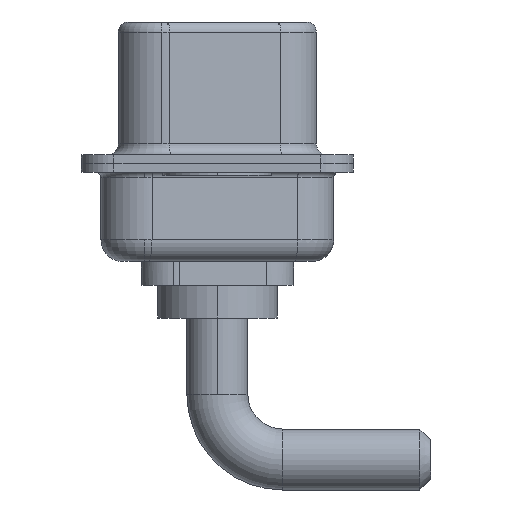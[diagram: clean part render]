
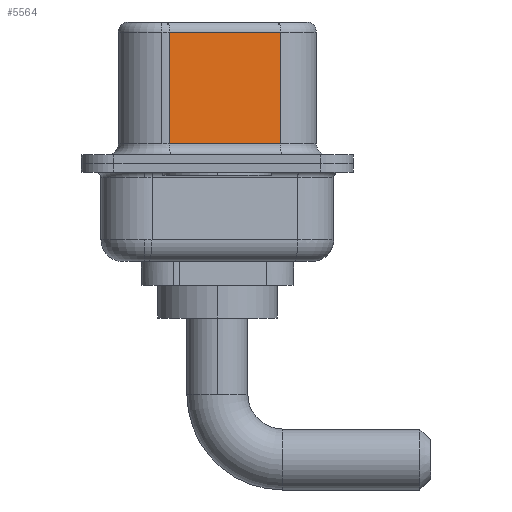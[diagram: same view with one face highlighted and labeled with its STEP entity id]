
A CAD part, left-side view. The second image highlights one B-rep face of the part: STEP entity #5564.
In plain terms, the highlighted planar face has unit normal (-0.985, -0.174, 0).
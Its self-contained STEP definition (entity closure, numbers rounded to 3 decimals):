
#86 = VECTOR ( 'NONE', #13597, 1000. ) ;
#564 = CARTESIAN_POINT ( 'NONE',  ( 3.68, 2.203, 6.02 ) ) ;
#1010 = DIRECTION ( 'NONE',  ( 0.174, -0.985, 0. ) ) ;
#1036 = EDGE_LOOP ( 'NONE', ( #1470, #6937, #10099, #8384 ) ) ;
#1463 = FACE_OUTER_BOUND ( 'NONE', #1036, .T. ) ;
#1470 = ORIENTED_EDGE ( 'NONE', *, *, #13379, .F. ) ;
#1583 = LINE ( 'NONE', #5954, #86 ) ;
#2079 = VECTOR ( 'NONE', #6700, 1000. ) ;
#2290 = CARTESIAN_POINT ( 'NONE',  ( 4.58, -2.897, 0.9 ) ) ;
#2529 = CARTESIAN_POINT ( 'NONE',  ( 4.58, -2.897, 6.52 ) ) ;
#2664 = LINE ( 'NONE', #5741, #14234 ) ;
#2770 = EDGE_CURVE ( 'NONE', #6604, #4736, #1583, .T. ) ;
#3302 = LINE ( 'NONE', #2290, #7508 ) ;
#3891 = EDGE_CURVE ( 'NONE', #5021, #6604, #4998, .T. ) ;
#4736 = VERTEX_POINT ( 'NONE', #10862 ) ;
#4998 = LINE ( 'NONE', #13854, #2079 ) ;
#5021 = VERTEX_POINT ( 'NONE', #9100 ) ;
#5564 = ADVANCED_FACE ( 'NONE', ( #1463 ), #5755, .F. ) ;
#5741 = CARTESIAN_POINT ( 'NONE',  ( 4.58, -2.897, 6.52 ) ) ;
#5755 = PLANE ( 'NONE',  #11990 ) ;
#5835 = DIRECTION ( 'NONE',  ( 0.985, 0.174, 0. ) ) ;
#5954 = CARTESIAN_POINT ( 'NONE',  ( 3.68, 2.203, 6.52 ) ) ;
#6604 = VERTEX_POINT ( 'NONE', #564 ) ;
#6700 = DIRECTION ( 'NONE',  ( -0.174, 0.985, 0. ) ) ;
#6937 = ORIENTED_EDGE ( 'NONE', *, *, #3891, .T. ) ;
#7508 = VECTOR ( 'NONE', #1010, 1000. ) ;
#8384 = ORIENTED_EDGE ( 'NONE', *, *, #13764, .T. ) ;
#9100 = CARTESIAN_POINT ( 'NONE',  ( 4.58, -2.897, 6.02 ) ) ;
#10099 = ORIENTED_EDGE ( 'NONE', *, *, #2770, .T. ) ;
#10308 = DIRECTION ( 'NONE',  ( -0.174, 0.985, 0. ) ) ;
#10862 = CARTESIAN_POINT ( 'NONE',  ( 3.68, 2.203, 0.9 ) ) ;
#11990 = AXIS2_PLACEMENT_3D ( 'NONE', #2529, #5835, #10308 ) ;
#12591 = VERTEX_POINT ( 'NONE', #12611 ) ;
#12611 = CARTESIAN_POINT ( 'NONE',  ( 4.58, -2.897, 0.9 ) ) ;
#13379 = EDGE_CURVE ( 'NONE', #5021, #12591, #2664, .T. ) ;
#13530 = DIRECTION ( 'NONE',  ( 0., 0., -1. ) ) ;
#13597 = DIRECTION ( 'NONE',  ( 0., 0., -1. ) ) ;
#13764 = EDGE_CURVE ( 'NONE', #4736, #12591, #3302, .T. ) ;
#13854 = CARTESIAN_POINT ( 'NONE',  ( 4.58, -2.897, 6.02 ) ) ;
#14234 = VECTOR ( 'NONE', #13530, 1000. ) ;
